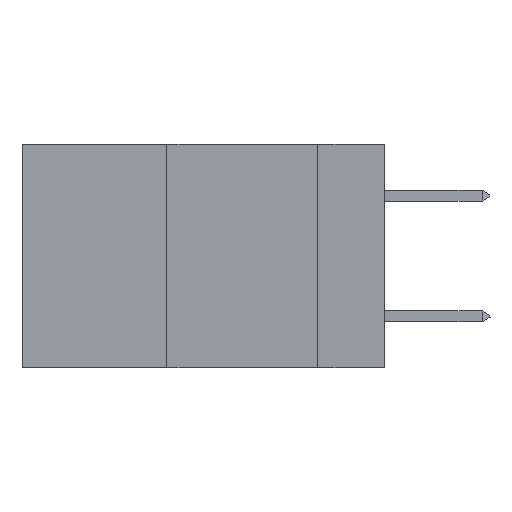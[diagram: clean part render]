
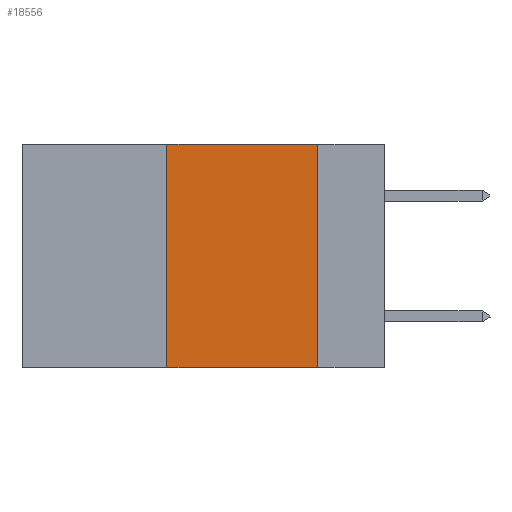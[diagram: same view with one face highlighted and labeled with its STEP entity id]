
A CAD part, left-side view. The second image highlights one B-rep face of the part: STEP entity #18556.
In plain terms, the highlighted planar face has unit normal (-1, 0, 0).
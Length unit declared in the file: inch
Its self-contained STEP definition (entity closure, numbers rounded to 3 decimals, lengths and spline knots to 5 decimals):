
#83 = CARTESIAN_POINT ( 'NONE',  ( 0., 0.36, -0.37 ) ) ;
#1294 = ORIENTED_EDGE ( 'NONE', *, *, #19558, .F. ) ;
#1900 = CARTESIAN_POINT ( 'NONE',  ( 0., 0.36, 0. ) ) ;
#2279 = VECTOR ( 'NONE', #13218, 39.37008 ) ;
#2339 = EDGE_LOOP ( 'NONE', ( #1294, #10365, #2875, #22979 ) ) ;
#2540 = CARTESIAN_POINT ( 'NONE',  ( 0., 0.11, 0. ) ) ;
#2875 = ORIENTED_EDGE ( 'NONE', *, *, #3014, .F. ) ;
#3014 = EDGE_CURVE ( 'NONE', #15781, #14054, #4011, .T. ) ;
#4011 = LINE ( 'NONE', #1900, #22480 ) ;
#4293 = CARTESIAN_POINT ( 'NONE',  ( 0., 0.6, 0. ) ) ;
#4499 = CARTESIAN_POINT ( 'NONE',  ( 0., 0.6, -0.37 ) ) ;
#6408 = VERTEX_POINT ( 'NONE', #6654 ) ;
#6654 = CARTESIAN_POINT ( 'NONE',  ( 0., 0.11, 0. ) ) ;
#7420 = CARTESIAN_POINT ( 'NONE',  ( 0., 0.11, -0.37 ) ) ;
#8636 = DIRECTION ( 'NONE',  ( 0., -1., 0. ) ) ;
#10365 = ORIENTED_EDGE ( 'NONE', *, *, #14851, .F. ) ;
#11246 = DIRECTION ( 'NONE',  ( 0., 0., -1. ) ) ;
#13218 = DIRECTION ( 'NONE',  ( 0., 0., -1. ) ) ;
#13392 = EDGE_CURVE ( 'NONE', #15781, #26947, #19389, .T. ) ;
#13631 = CARTESIAN_POINT ( 'NONE',  ( 0., 0.6, 0. ) ) ;
#14054 = VERTEX_POINT ( 'NONE', #18640 ) ;
#14851 = EDGE_CURVE ( 'NONE', #14054, #6408, #23549, .T. ) ;
#15781 = VERTEX_POINT ( 'NONE', #83 ) ;
#15863 = DIRECTION ( 'NONE',  ( 1., 0., 0. ) ) ;
#17279 = DIRECTION ( 'NONE',  ( 0., -1., 0. ) ) ;
#17552 = LINE ( 'NONE', #2540, #2279 ) ;
#18556 = ADVANCED_FACE ( 'NONE', ( #24466 ), #19943, .F. ) ;
#18640 = CARTESIAN_POINT ( 'NONE',  ( 0., 0.36, 0. ) ) ;
#19045 = DIRECTION ( 'NONE',  ( 0., 0., 1. ) ) ;
#19389 = LINE ( 'NONE', #4499, #23662 ) ;
#19558 = EDGE_CURVE ( 'NONE', #6408, #26947, #17552, .T. ) ;
#19943 = PLANE ( 'NONE',  #26946 ) ;
#22480 = VECTOR ( 'NONE', #19045, 39.37008 ) ;
#22979 = ORIENTED_EDGE ( 'NONE', *, *, #13392, .T. ) ;
#23549 = LINE ( 'NONE', #4293, #27755 ) ;
#23662 = VECTOR ( 'NONE', #17279, 39.37008 ) ;
#24466 = FACE_OUTER_BOUND ( 'NONE', #2339, .T. ) ;
#26946 = AXIS2_PLACEMENT_3D ( 'NONE', #13631, #15863, #11246 ) ;
#26947 = VERTEX_POINT ( 'NONE', #7420 ) ;
#27755 = VECTOR ( 'NONE', #8636, 39.37008 ) ;
